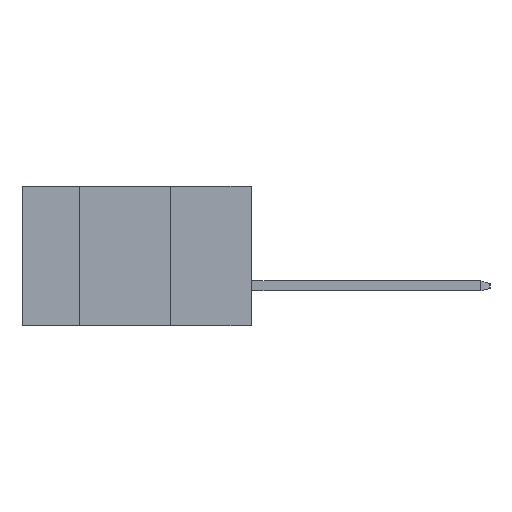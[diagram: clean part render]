
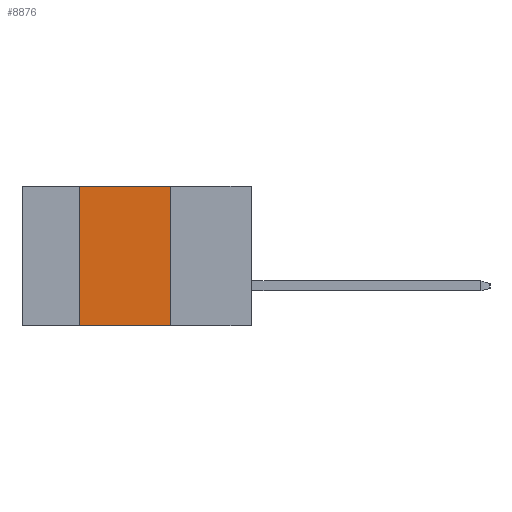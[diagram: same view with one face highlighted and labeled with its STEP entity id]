
A CAD part, left-side view. The second image highlights one B-rep face of the part: STEP entity #8876.
In plain terms, the highlighted planar face has unit normal (-1, 0, 0).
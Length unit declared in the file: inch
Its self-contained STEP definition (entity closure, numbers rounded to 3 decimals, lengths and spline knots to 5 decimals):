
#199 = VERTEX_POINT ( 'NONE', #6637 ) ;
#380 = DIRECTION ( 'NONE',  ( 1., 0., 0. ) ) ;
#1308 = DIRECTION ( 'NONE',  ( 0., -1., 0. ) ) ;
#1796 = CARTESIAN_POINT ( 'NONE',  ( 0., 0.254, -0.437 ) ) ;
#1866 = VECTOR ( 'NONE', #6059, 39.37008 ) ;
#2137 = DIRECTION ( 'NONE',  ( 0., 0., -1. ) ) ;
#2579 = EDGE_CURVE ( 'NONE', #2597, #4921, #8744, .T. ) ;
#2597 = VERTEX_POINT ( 'NONE', #8140 ) ;
#2675 = AXIS2_PLACEMENT_3D ( 'NONE', #3969, #380, #5972 ) ;
#2734 = ORIENTED_EDGE ( 'NONE', *, *, #2579, .F. ) ;
#3234 = ORIENTED_EDGE ( 'NONE', *, *, #8964, .T. ) ;
#3392 = LINE ( 'NONE', #6827, #3835 ) ;
#3507 = LINE ( 'NONE', #6280, #7244 ) ;
#3730 = VERTEX_POINT ( 'NONE', #1796 ) ;
#3835 = VECTOR ( 'NONE', #4879, 39.37008 ) ;
#3969 = CARTESIAN_POINT ( 'NONE',  ( 0., 0.72, 0. ) ) ;
#4164 = ORIENTED_EDGE ( 'NONE', *, *, #8062, .F. ) ;
#4213 = ORIENTED_EDGE ( 'NONE', *, *, #6514, .F. ) ;
#4422 = EDGE_LOOP ( 'NONE', ( #4213, #4164, #2734, #3234 ) ) ;
#4687 = VECTOR ( 'NONE', #1308, 39.37008 ) ;
#4879 = DIRECTION ( 'NONE',  ( 0., -1., 0. ) ) ;
#4921 = VERTEX_POINT ( 'NONE', #7682 ) ;
#5972 = DIRECTION ( 'NONE',  ( 0., 0., -1. ) ) ;
#6059 = DIRECTION ( 'NONE',  ( 0., 0., 1. ) ) ;
#6105 = FACE_OUTER_BOUND ( 'NONE', #4422, .T. ) ;
#6107 = CARTESIAN_POINT ( 'NONE',  ( 0., 0.54, -0.437 ) ) ;
#6280 = CARTESIAN_POINT ( 'NONE',  ( 0., 0.254, -0.437 ) ) ;
#6514 = EDGE_CURVE ( 'NONE', #199, #3730, #3507, .T. ) ;
#6637 = CARTESIAN_POINT ( 'NONE',  ( 0., 0.254, 0. ) ) ;
#6776 = PLANE ( 'NONE',  #2675 ) ;
#6827 = CARTESIAN_POINT ( 'NONE',  ( 0., 0.72, -0.437 ) ) ;
#7244 = VECTOR ( 'NONE', #2137, 39.37008 ) ;
#7517 = LINE ( 'NONE', #8897, #4687 ) ;
#7682 = CARTESIAN_POINT ( 'NONE',  ( 0., 0.54, 0. ) ) ;
#8062 = EDGE_CURVE ( 'NONE', #4921, #199, #7517, .T. ) ;
#8140 = CARTESIAN_POINT ( 'NONE',  ( 0., 0.54, -0.437 ) ) ;
#8744 = LINE ( 'NONE', #6107, #1866 ) ;
#8876 = ADVANCED_FACE ( 'NONE', ( #6105 ), #6776, .F. ) ;
#8897 = CARTESIAN_POINT ( 'NONE',  ( 0., 0.72, 0. ) ) ;
#8964 = EDGE_CURVE ( 'NONE', #2597, #3730, #3392, .T. ) ;
